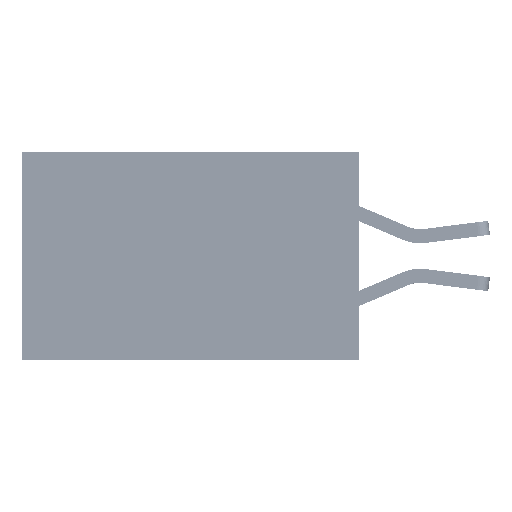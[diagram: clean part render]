
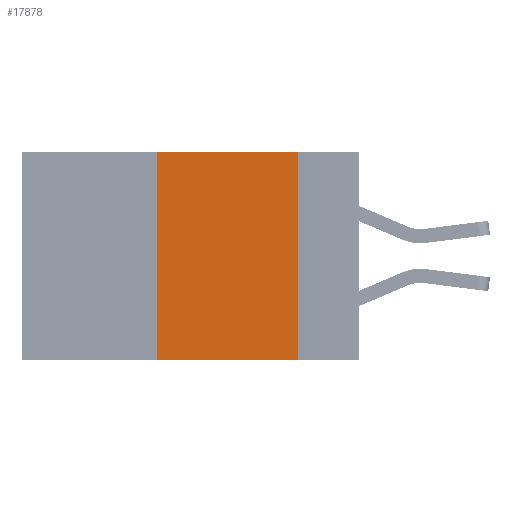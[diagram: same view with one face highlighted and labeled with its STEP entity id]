
A CAD part, left-side view. The second image highlights one B-rep face of the part: STEP entity #17878.
In plain terms, the highlighted planar face has unit normal (-1, 0, 0).
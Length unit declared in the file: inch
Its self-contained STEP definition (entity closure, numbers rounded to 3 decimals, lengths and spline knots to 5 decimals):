
#653 = CARTESIAN_POINT ( 'NONE',  ( 0., 0.6, -0.37 ) ) ;
#942 = CARTESIAN_POINT ( 'NONE',  ( 0., 0.6, 0. ) ) ;
#1726 = DIRECTION ( 'NONE',  ( 0., 0., 1. ) ) ;
#2849 = CARTESIAN_POINT ( 'NONE',  ( 0., 0.36, 0. ) ) ;
#5015 = CARTESIAN_POINT ( 'NONE',  ( 0., 0.6, 0. ) ) ;
#5451 = VERTEX_POINT ( 'NONE', #33548 ) ;
#5606 = EDGE_CURVE ( 'NONE', #19903, #16040, #17959, .T. ) ;
#7676 = DIRECTION ( 'NONE',  ( 0., -1., 0. ) ) ;
#10425 = VECTOR ( 'NONE', #18417, 39.37008 ) ;
#10774 = ORIENTED_EDGE ( 'NONE', *, *, #30598, .T. ) ;
#11491 = LINE ( 'NONE', #942, #10425 ) ;
#11827 = LINE ( 'NONE', #20526, #35186 ) ;
#12625 = DIRECTION ( 'NONE',  ( 1., 0., 0. ) ) ;
#16040 = VERTEX_POINT ( 'NONE', #29998 ) ;
#17574 = FACE_OUTER_BOUND ( 'NONE', #23038, .T. ) ;
#17878 = ADVANCED_FACE ( 'NONE', ( #17574 ), #32823, .F. ) ;
#17959 = LINE ( 'NONE', #2849, #37533 ) ;
#18417 = DIRECTION ( 'NONE',  ( 0., -1., 0. ) ) ;
#19075 = ORIENTED_EDGE ( 'NONE', *, *, #5606, .F. ) ;
#19903 = VERTEX_POINT ( 'NONE', #40833 ) ;
#20526 = CARTESIAN_POINT ( 'NONE',  ( 0., 0.11, 0. ) ) ;
#22964 = VECTOR ( 'NONE', #7676, 39.37008 ) ;
#23038 = EDGE_LOOP ( 'NONE', ( #29071, #33249, #19075, #10774 ) ) ;
#23952 = EDGE_CURVE ( 'NONE', #16040, #5451, #11491, .T. ) ;
#25867 = DIRECTION ( 'NONE',  ( 0., 0., -1. ) ) ;
#26773 = LINE ( 'NONE', #653, #22964 ) ;
#29071 = ORIENTED_EDGE ( 'NONE', *, *, #42609, .F. ) ;
#29998 = CARTESIAN_POINT ( 'NONE',  ( 0., 0.36, 0. ) ) ;
#30598 = EDGE_CURVE ( 'NONE', #19903, #37386, #26773, .T. ) ;
#32823 = PLANE ( 'NONE',  #44263 ) ;
#33249 = ORIENTED_EDGE ( 'NONE', *, *, #23952, .F. ) ;
#33548 = CARTESIAN_POINT ( 'NONE',  ( 0., 0.11, 0. ) ) ;
#35186 = VECTOR ( 'NONE', #44853, 39.37008 ) ;
#37386 = VERTEX_POINT ( 'NONE', #43215 ) ;
#37533 = VECTOR ( 'NONE', #1726, 39.37008 ) ;
#40833 = CARTESIAN_POINT ( 'NONE',  ( 0., 0.36, -0.37 ) ) ;
#42609 = EDGE_CURVE ( 'NONE', #5451, #37386, #11827, .T. ) ;
#43215 = CARTESIAN_POINT ( 'NONE',  ( 0., 0.11, -0.37 ) ) ;
#44263 = AXIS2_PLACEMENT_3D ( 'NONE', #5015, #12625, #25867 ) ;
#44853 = DIRECTION ( 'NONE',  ( 0., 0., -1. ) ) ;
